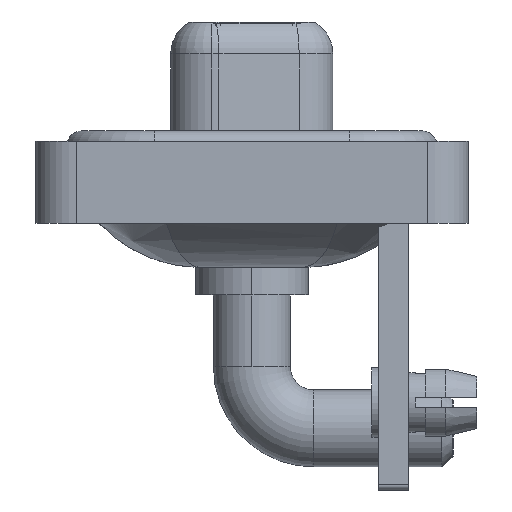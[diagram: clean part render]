
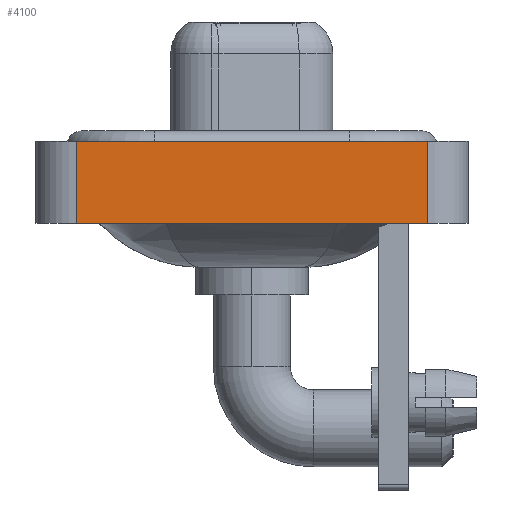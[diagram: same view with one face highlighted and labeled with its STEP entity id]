
A CAD part, left-side view. The second image highlights one B-rep face of the part: STEP entity #4100.
In plain terms, the highlighted planar face has unit normal (-1, 0, 0).
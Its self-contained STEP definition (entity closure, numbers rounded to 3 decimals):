
#511 = LINE ( 'NONE', #16256, #1215 ) ;
#1215 = VECTOR ( 'NONE', #2501, 1000. ) ;
#1271 = ORIENTED_EDGE ( 'NONE', *, *, #18061, .T. ) ;
#1323 = LINE ( 'NONE', #7850, #18560 ) ;
#1360 = CARTESIAN_POINT ( 'NONE',  ( -7.3, -8.55, -3.6 ) ) ;
#1367 = VERTEX_POINT ( 'NONE', #12138 ) ;
#1850 = CARTESIAN_POINT ( 'NONE',  ( -7.3, -8.55, -3.6 ) ) ;
#2376 = LINE ( 'NONE', #19071, #8961 ) ;
#2501 = DIRECTION ( 'NONE',  ( 0., -1., 0. ) ) ;
#3552 = AXIS2_PLACEMENT_3D ( 'NONE', #13486, #4541, #15364 ) ;
#4100 = ADVANCED_FACE ( 'NONE', ( #12074 ), #10758, .T. ) ;
#4541 = DIRECTION ( 'NONE',  ( -1., 0., 0. ) ) ;
#5148 = CARTESIAN_POINT ( 'NONE',  ( -7.3, -8.55, 0.4 ) ) ;
#7207 = VERTEX_POINT ( 'NONE', #10255 ) ;
#7850 = CARTESIAN_POINT ( 'NONE',  ( -7.3, -8.55, 0.4 ) ) ;
#8504 = DIRECTION ( 'NONE',  ( 0., 0., 1. ) ) ;
#8837 = VERTEX_POINT ( 'NONE', #1360 ) ;
#8961 = VECTOR ( 'NONE', #8504, 1000. ) ;
#10255 = CARTESIAN_POINT ( 'NONE',  ( -7.3, 8.55, 0.4 ) ) ;
#10758 = PLANE ( 'NONE',  #3552 ) ;
#12048 = EDGE_LOOP ( 'NONE', ( #1271, #12149, #18978, #19351 ) ) ;
#12074 = FACE_OUTER_BOUND ( 'NONE', #12048, .T. ) ;
#12138 = CARTESIAN_POINT ( 'NONE',  ( -7.3, 8.55, -3.6 ) ) ;
#12149 = ORIENTED_EDGE ( 'NONE', *, *, #17234, .F. ) ;
#12610 = LINE ( 'NONE', #1850, #17963 ) ;
#13486 = CARTESIAN_POINT ( 'NONE',  ( -7.3, -8.55, -3.6 ) ) ;
#13962 = DIRECTION ( 'NONE',  ( 0., -1., 0. ) ) ;
#15364 = DIRECTION ( 'NONE',  ( 0., 0., 1. ) ) ;
#16256 = CARTESIAN_POINT ( 'NONE',  ( -7.3, -8.55, -3.6 ) ) ;
#16428 = EDGE_CURVE ( 'NONE', #1367, #7207, #2376, .T. ) ;
#17234 = EDGE_CURVE ( 'NONE', #7207, #17407, #1323, .T. ) ;
#17357 = EDGE_CURVE ( 'NONE', #1367, #8837, #511, .T. ) ;
#17407 = VERTEX_POINT ( 'NONE', #5148 ) ;
#17963 = VECTOR ( 'NONE', #18539, 1000. ) ;
#18061 = EDGE_CURVE ( 'NONE', #8837, #17407, #12610, .T. ) ;
#18539 = DIRECTION ( 'NONE',  ( 0., 0., 1. ) ) ;
#18560 = VECTOR ( 'NONE', #13962, 1000. ) ;
#18978 = ORIENTED_EDGE ( 'NONE', *, *, #16428, .F. ) ;
#19071 = CARTESIAN_POINT ( 'NONE',  ( -7.3, 8.55, -3.6 ) ) ;
#19351 = ORIENTED_EDGE ( 'NONE', *, *, #17357, .T. ) ;
